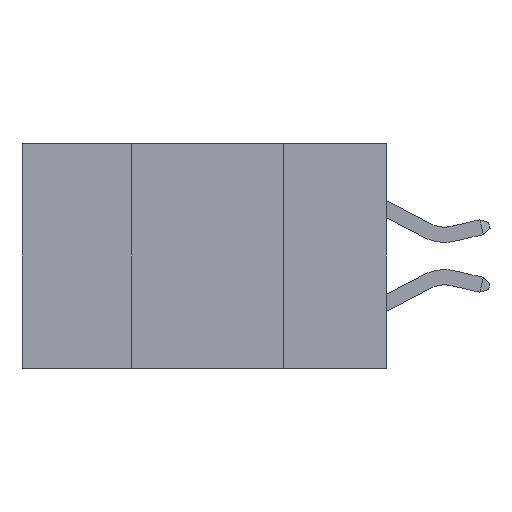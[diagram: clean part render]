
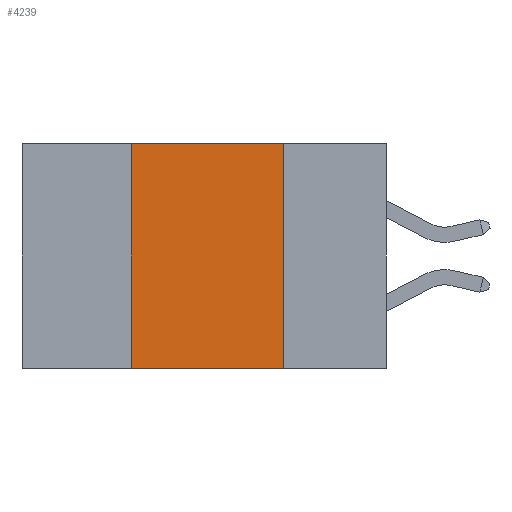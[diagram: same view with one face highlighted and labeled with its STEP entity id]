
A CAD part, left-side view. The second image highlights one B-rep face of the part: STEP entity #4239.
In plain terms, the highlighted planar face has unit normal (-1, 0, 0).
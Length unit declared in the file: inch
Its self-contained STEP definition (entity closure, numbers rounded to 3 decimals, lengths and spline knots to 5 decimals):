
#33 = ORIENTED_EDGE ( 'NONE', *, *, #6462, .F. ) ;
#1922 = EDGE_CURVE ( 'NONE', #15012, #13267, #25754, .T. ) ;
#2324 = DIRECTION ( 'NONE',  ( 0., 0., 1. ) ) ;
#3952 = CARTESIAN_POINT ( 'NONE',  ( 0., 0.42, -0.37 ) ) ;
#4239 = ADVANCED_FACE ( 'NONE', ( #24906 ), #21083, .F. ) ;
#4353 = EDGE_CURVE ( 'NONE', #25261, #15012, #25821, .T. ) ;
#4837 = LINE ( 'NONE', #24873, #13084 ) ;
#6070 = EDGE_CURVE ( 'NONE', #8173, #13267, #4837, .T. ) ;
#6462 = EDGE_CURVE ( 'NONE', #8173, #25261, #12288, .T. ) ;
#6880 = CARTESIAN_POINT ( 'NONE',  ( 0., 0.17, 0. ) ) ;
#7823 = CARTESIAN_POINT ( 'NONE',  ( 0., 0.17, -0.37 ) ) ;
#8173 = VERTEX_POINT ( 'NONE', #3952 ) ;
#9204 = CARTESIAN_POINT ( 'NONE',  ( 0., 0.6, 0. ) ) ;
#10070 = ORIENTED_EDGE ( 'NONE', *, *, #6070, .T. ) ;
#10313 = CARTESIAN_POINT ( 'NONE',  ( 0., 0.17, -0.37 ) ) ;
#10495 = VECTOR ( 'NONE', #19704, 39.37008 ) ;
#10607 = ORIENTED_EDGE ( 'NONE', *, *, #1922, .F. ) ;
#12288 = LINE ( 'NONE', #20263, #15570 ) ;
#12649 = CARTESIAN_POINT ( 'NONE',  ( 0., 0.42, 0. ) ) ;
#12967 = DIRECTION ( 'NONE',  ( 0., -1., 0. ) ) ;
#13084 = VECTOR ( 'NONE', #12967, 39.37008 ) ;
#13267 = VERTEX_POINT ( 'NONE', #10313 ) ;
#13868 = CARTESIAN_POINT ( 'NONE',  ( 0., 0.6, 0. ) ) ;
#15012 = VERTEX_POINT ( 'NONE', #6880 ) ;
#15179 = DIRECTION ( 'NONE',  ( 0., 0., -1. ) ) ;
#15570 = VECTOR ( 'NONE', #2324, 39.37008 ) ;
#19704 = DIRECTION ( 'NONE',  ( 0., 0., -1. ) ) ;
#19767 = VECTOR ( 'NONE', #23712, 39.37008 ) ;
#20263 = CARTESIAN_POINT ( 'NONE',  ( 0., 0.42, -0.37 ) ) ;
#21083 = PLANE ( 'NONE',  #21409 ) ;
#21409 = AXIS2_PLACEMENT_3D ( 'NONE', #9204, #24778, #15179 ) ;
#23258 = ORIENTED_EDGE ( 'NONE', *, *, #4353, .F. ) ;
#23286 = EDGE_LOOP ( 'NONE', ( #10607, #23258, #33, #10070 ) ) ;
#23712 = DIRECTION ( 'NONE',  ( 0., -1., 0. ) ) ;
#24778 = DIRECTION ( 'NONE',  ( 1., 0., 0. ) ) ;
#24873 = CARTESIAN_POINT ( 'NONE',  ( 0., 0.6, -0.37 ) ) ;
#24906 = FACE_OUTER_BOUND ( 'NONE', #23286, .T. ) ;
#25261 = VERTEX_POINT ( 'NONE', #12649 ) ;
#25754 = LINE ( 'NONE', #7823, #10495 ) ;
#25821 = LINE ( 'NONE', #13868, #19767 ) ;
